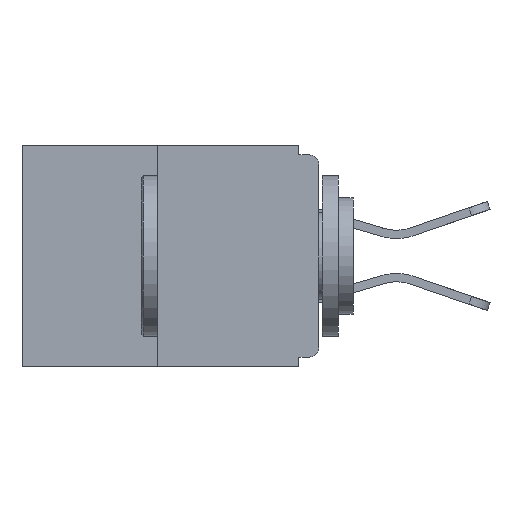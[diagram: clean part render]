
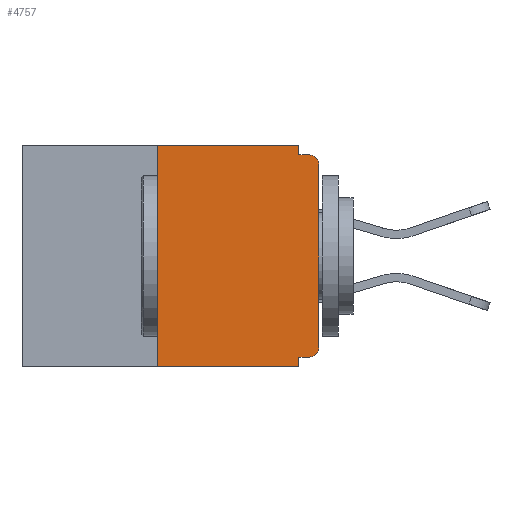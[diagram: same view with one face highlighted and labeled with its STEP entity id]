
A CAD part, left-side view. The second image highlights one B-rep face of the part: STEP entity #4757.
In plain terms, the highlighted planar face has unit normal (-1, 0, 0).
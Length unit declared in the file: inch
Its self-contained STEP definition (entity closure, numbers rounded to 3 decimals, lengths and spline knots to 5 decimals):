
#926 = CARTESIAN_POINT ( 'NONE',  ( 0., 0.46, 0. ) ) ;
#1000 = VECTOR ( 'NONE', #6182, 39.37008 ) ;
#1486 = AXIS2_PLACEMENT_3D ( 'NONE', #18636, #23584, #11015 ) ;
#1730 = VERTEX_POINT ( 'NONE', #26288 ) ;
#1777 = VERTEX_POINT ( 'NONE', #28970 ) ;
#2682 = CARTESIAN_POINT ( 'NONE',  ( 0., 0.031, -0.015 ) ) ;
#3108 = LINE ( 'NONE', #16609, #27261 ) ;
#3832 = DIRECTION ( 'NONE',  ( 0., -1., 0. ) ) ;
#4752 = CARTESIAN_POINT ( 'NONE',  ( 0., 0.015, -0.328 ) ) ;
#4757 = ADVANCED_FACE ( 'NONE', ( #11468 ), #31181, .F. ) ;
#5452 = ORIENTED_EDGE ( 'NONE', *, *, #13511, .T. ) ;
#6182 = DIRECTION ( 'NONE',  ( 0., -1., 0. ) ) ;
#6289 = CARTESIAN_POINT ( 'NONE',  ( 0., 0.46, 0. ) ) ;
#6333 = EDGE_CURVE ( 'NONE', #16382, #14952, #22234, .T. ) ;
#7728 = CARTESIAN_POINT ( 'NONE',  ( 0., 0., -0.015 ) ) ;
#8193 = DIRECTION ( 'NONE',  ( 1., 0., 0. ) ) ;
#8226 = CARTESIAN_POINT ( 'NONE',  ( 0., 0.031, -0.328 ) ) ;
#8700 = CARTESIAN_POINT ( 'NONE',  ( 0., 0.46, -0.343 ) ) ;
#8797 = CARTESIAN_POINT ( 'NONE',  ( 0., 0.015, -0.015 ) ) ;
#9018 = VECTOR ( 'NONE', #18339, 39.37008 ) ;
#9938 = EDGE_CURVE ( 'NONE', #1730, #11217, #32025, .T. ) ;
#10249 = VECTOR ( 'NONE', #3832, 39.37008 ) ;
#10300 = VERTEX_POINT ( 'NONE', #27008 ) ;
#11015 = DIRECTION ( 'NONE',  ( 0., 0., -1. ) ) ;
#11217 = VERTEX_POINT ( 'NONE', #8797 ) ;
#11468 = FACE_OUTER_BOUND ( 'NONE', #16784, .T. ) ;
#11664 = VERTEX_POINT ( 'NONE', #26648 ) ;
#11710 = CARTESIAN_POINT ( 'NONE',  ( 0., 0.25, 0. ) ) ;
#12243 = LINE ( 'NONE', #8700, #10249 ) ;
#12485 = EDGE_CURVE ( 'NONE', #16382, #11664, #17242, .T. ) ;
#13112 = EDGE_CURVE ( 'NONE', #10300, #21549, #21104, .T. ) ;
#13511 = EDGE_CURVE ( 'NONE', #19589, #1777, #12243, .T. ) ;
#13516 = LINE ( 'NONE', #30417, #23783 ) ;
#14198 = EDGE_CURVE ( 'NONE', #11664, #1730, #24026, .T. ) ;
#14233 = CARTESIAN_POINT ( 'NONE',  ( 0., 0.031, 0. ) ) ;
#14428 = LINE ( 'NONE', #6289, #1000 ) ;
#14922 = DIRECTION ( 'NONE',  ( 0., -1., 0. ) ) ;
#14925 = DIRECTION ( 'NONE',  ( 0., 0., 1. ) ) ;
#14952 = VERTEX_POINT ( 'NONE', #8226 ) ;
#15461 = AXIS2_PLACEMENT_3D ( 'NONE', #926, #8193, #31302 ) ;
#15558 = EDGE_CURVE ( 'NONE', #28133, #10300, #14428, .T. ) ;
#15875 = VECTOR ( 'NONE', #27305, 39.37008 ) ;
#15930 = ORIENTED_EDGE ( 'NONE', *, *, #31685, .F. ) ;
#15951 = LINE ( 'NONE', #7728, #25851 ) ;
#16089 = CARTESIAN_POINT ( 'NONE',  ( 0., 0., 0. ) ) ;
#16332 = EDGE_CURVE ( 'NONE', #21549, #11217, #15951, .T. ) ;
#16382 = VERTEX_POINT ( 'NONE', #4752 ) ;
#16597 = DIRECTION ( 'NONE',  ( 0., 0., -1. ) ) ;
#16609 = CARTESIAN_POINT ( 'NONE',  ( 0., 0.031, -0.343 ) ) ;
#16784 = EDGE_LOOP ( 'NONE', ( #24270, #21698, #5452, #15930, #17990, #18771, #25463, #28153, #17338, #31611 ) ) ;
#17242 = CIRCLE ( 'NONE', #1486, 0.015 ) ;
#17338 = ORIENTED_EDGE ( 'NONE', *, *, #16332, .F. ) ;
#17393 = VECTOR ( 'NONE', #28968, 39.37008 ) ;
#17990 = ORIENTED_EDGE ( 'NONE', *, *, #6333, .F. ) ;
#18339 = DIRECTION ( 'NONE',  ( 0., 0., 1. ) ) ;
#18636 = CARTESIAN_POINT ( 'NONE',  ( 0., 0.015, -0.313 ) ) ;
#18771 = ORIENTED_EDGE ( 'NONE', *, *, #12485, .T. ) ;
#18936 = DIRECTION ( 'NONE',  ( -1., 0., 0. ) ) ;
#19589 = VERTEX_POINT ( 'NONE', #21283 ) ;
#21104 = LINE ( 'NONE', #14233, #17393 ) ;
#21283 = CARTESIAN_POINT ( 'NONE',  ( 0., 0.25, -0.343 ) ) ;
#21549 = VERTEX_POINT ( 'NONE', #2682 ) ;
#21698 = ORIENTED_EDGE ( 'NONE', *, *, #27708, .F. ) ;
#22234 = LINE ( 'NONE', #26862, #15875 ) ;
#22982 = AXIS2_PLACEMENT_3D ( 'NONE', #31740, #18936, #16597 ) ;
#23584 = DIRECTION ( 'NONE',  ( -1., 0., 0. ) ) ;
#23783 = VECTOR ( 'NONE', #14925, 39.37008 ) ;
#24026 = LINE ( 'NONE', #16089, #9018 ) ;
#24108 = DIRECTION ( 'NONE',  ( 0., 0., -1. ) ) ;
#24270 = ORIENTED_EDGE ( 'NONE', *, *, #15558, .F. ) ;
#25463 = ORIENTED_EDGE ( 'NONE', *, *, #14198, .T. ) ;
#25851 = VECTOR ( 'NONE', #14922, 39.37008 ) ;
#26288 = CARTESIAN_POINT ( 'NONE',  ( 0., 0., -0.03 ) ) ;
#26648 = CARTESIAN_POINT ( 'NONE',  ( 0., 0., -0.313 ) ) ;
#26862 = CARTESIAN_POINT ( 'NONE',  ( 0., 0., -0.328 ) ) ;
#27008 = CARTESIAN_POINT ( 'NONE',  ( 0., 0.031, 0. ) ) ;
#27261 = VECTOR ( 'NONE', #24108, 39.37008 ) ;
#27305 = DIRECTION ( 'NONE',  ( 0., 1., 0. ) ) ;
#27708 = EDGE_CURVE ( 'NONE', #19589, #28133, #13516, .T. ) ;
#28133 = VERTEX_POINT ( 'NONE', #11710 ) ;
#28153 = ORIENTED_EDGE ( 'NONE', *, *, #9938, .T. ) ;
#28968 = DIRECTION ( 'NONE',  ( 0., 0., -1. ) ) ;
#28970 = CARTESIAN_POINT ( 'NONE',  ( 0., 0.031, -0.343 ) ) ;
#30417 = CARTESIAN_POINT ( 'NONE',  ( 0., 0.25, 0. ) ) ;
#31181 = PLANE ( 'NONE',  #15461 ) ;
#31302 = DIRECTION ( 'NONE',  ( 0., 0., -1. ) ) ;
#31611 = ORIENTED_EDGE ( 'NONE', *, *, #13112, .F. ) ;
#31685 = EDGE_CURVE ( 'NONE', #14952, #1777, #3108, .T. ) ;
#31740 = CARTESIAN_POINT ( 'NONE',  ( 0., 0.015, -0.03 ) ) ;
#32025 = CIRCLE ( 'NONE', #22982, 0.015 ) ;
